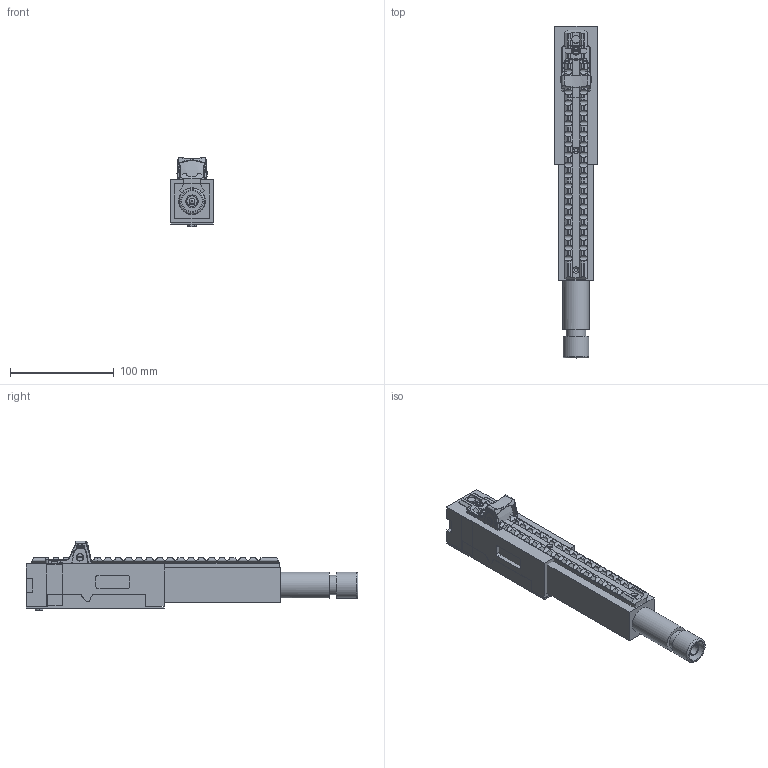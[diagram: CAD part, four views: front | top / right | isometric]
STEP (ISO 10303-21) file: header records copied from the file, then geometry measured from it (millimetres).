
FILE_DESCRIPTION(/* description */ (''),/* implementation_level */ '2;1');
FILE_NAME(/* name */ 'JIG DBMkCarbon.step',/* time_stamp */ '2022-05-18T14:12:38-07:00',/* author */ (''),/* organization */ (''),/* preprocessor_version */ 'ST-DEVELOPER v18.1',/* originating_system */ 'Autodesk Translation Framework v10.14.0.1471',/* authorisation */ '');
FILE_SCHEMA (('AUTOMOTIVE_DESIGN { 1 0 10303 214 3 1 1 }'));
Products named in the file (6): JIG DBMkCarbon; Barrel-Plug; Muzzle Plug (1); Short Rail; Long Rail; RMR
Assembly tree (5 placements, depth 2):
  JIG DBMkCarbon
    Barrel-Plug
    Muzzle Plug (1)
    Short Rail
    Long Rail
    RMR
Bounding box: 41 x 319.8 x 66.7 mm (x, y, z)
Volume: 550934.4 mm3; surface area: 219197.7 mm2
Topology: 14 solids, 15 shells, 2129 faces, 5719 edges, 3707 vertices
Faces by surface type: plane 896, cylinder 582, bspline 565, torus 45, sphere 22, cone 19
Full cylindrical faces by diameter (mm): 2.9 x1, 3 x9, 3.5 x12, 4 x7, 5.5 x1, 5.537 x2, 6 x9, 6.2 x2, 6.5 x2, 7 x2, 7.15 x2, 7.85 x2, 10.2 x1, 10.3 x1, 12.1 x1, 18.6 x1, 18.8 x1, 18.85 x1, 19.05 x1, 20 x1, 25 x1, 25.4 x1, 25.7 x4
Entity records: 99478 total; most frequent: CARTESIAN_POINT 49618, ORIENTED_EDGE 11414, DIRECTION 8704, EDGE_CURVE 5707, VERTEX_POINT 3707, AXIS2_PLACEMENT_3D 2925, LINE 2854, VECTOR 2854
